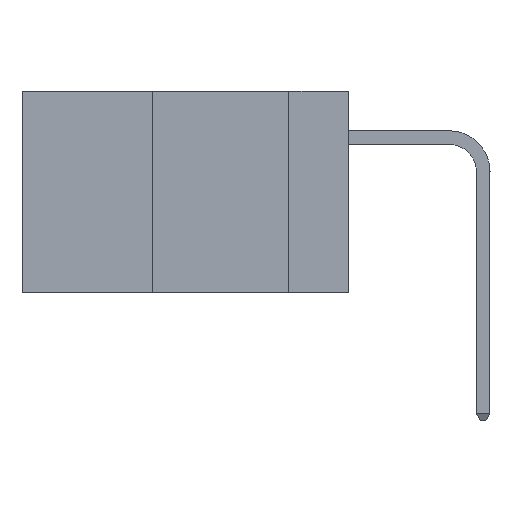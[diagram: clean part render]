
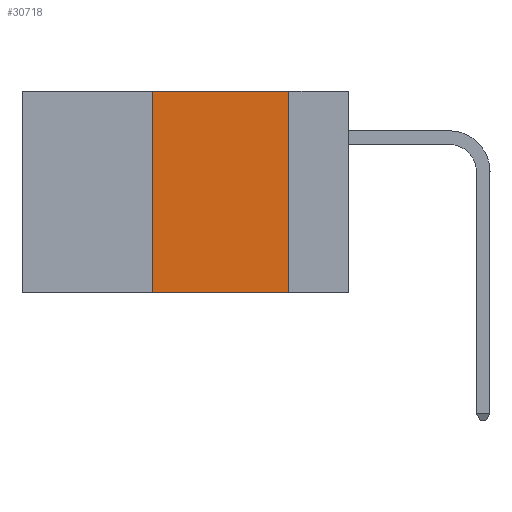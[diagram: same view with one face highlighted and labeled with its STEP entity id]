
A CAD part, left-side view. The second image highlights one B-rep face of the part: STEP entity #30718.
In plain terms, the highlighted planar face has unit normal (-1, 0, 0).
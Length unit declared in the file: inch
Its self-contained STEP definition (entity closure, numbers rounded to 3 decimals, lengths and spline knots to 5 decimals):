
#82 = CARTESIAN_POINT ( 'NONE',  ( 0., 0.11, 0. ) ) ;
#276 = DIRECTION ( 'NONE',  ( 0., 0., 1. ) ) ;
#2072 = CARTESIAN_POINT ( 'NONE',  ( 0., 0.11, 0. ) ) ;
#4077 = CARTESIAN_POINT ( 'NONE',  ( 0., 0.6, 0. ) ) ;
#4151 = ORIENTED_EDGE ( 'NONE', *, *, #21956, .F. ) ;
#4376 = CARTESIAN_POINT ( 'NONE',  ( 0., 0.6, -0.37 ) ) ;
#4894 = ORIENTED_EDGE ( 'NONE', *, *, #28098, .F. ) ;
#7425 = CARTESIAN_POINT ( 'NONE',  ( 0., 0.36, -0.37 ) ) ;
#9056 = DIRECTION ( 'NONE',  ( 0., 0., -1. ) ) ;
#9481 = CARTESIAN_POINT ( 'NONE',  ( 0., 0.6, 0. ) ) ;
#11064 = LINE ( 'NONE', #4077, #31831 ) ;
#12893 = ORIENTED_EDGE ( 'NONE', *, *, #17279, .T. ) ;
#13644 = VECTOR ( 'NONE', #29639, 39.37008 ) ;
#16273 = LINE ( 'NONE', #2072, #13644 ) ;
#17200 = DIRECTION ( 'NONE',  ( 0., -1., 0. ) ) ;
#17279 = EDGE_CURVE ( 'NONE', #19058, #21318, #33983, .T. ) ;
#17374 = VECTOR ( 'NONE', #276, 39.37008 ) ;
#18707 = VERTEX_POINT ( 'NONE', #35696 ) ;
#19058 = VERTEX_POINT ( 'NONE', #7425 ) ;
#21318 = VERTEX_POINT ( 'NONE', #23985 ) ;
#21956 = EDGE_CURVE ( 'NONE', #18707, #43145, #11064, .T. ) ;
#22112 = EDGE_CURVE ( 'NONE', #19058, #18707, #24281, .T. ) ;
#23985 = CARTESIAN_POINT ( 'NONE',  ( 0., 0.11, -0.37 ) ) ;
#24281 = LINE ( 'NONE', #31182, #17374 ) ;
#26159 = DIRECTION ( 'NONE',  ( 1., 0., 0. ) ) ;
#26860 = AXIS2_PLACEMENT_3D ( 'NONE', #9481, #26159, #9056 ) ;
#26951 = ORIENTED_EDGE ( 'NONE', *, *, #22112, .F. ) ;
#28098 = EDGE_CURVE ( 'NONE', #43145, #21318, #16273, .T. ) ;
#28211 = DIRECTION ( 'NONE',  ( 0., -1., 0. ) ) ;
#29639 = DIRECTION ( 'NONE',  ( 0., 0., -1. ) ) ;
#30718 = ADVANCED_FACE ( 'NONE', ( #34786 ), #42939, .F. ) ;
#31182 = CARTESIAN_POINT ( 'NONE',  ( 0., 0.36, 0. ) ) ;
#31831 = VECTOR ( 'NONE', #17200, 39.37008 ) ;
#33983 = LINE ( 'NONE', #4376, #43523 ) ;
#34786 = FACE_OUTER_BOUND ( 'NONE', #36191, .T. ) ;
#35696 = CARTESIAN_POINT ( 'NONE',  ( 0., 0.36, 0. ) ) ;
#36191 = EDGE_LOOP ( 'NONE', ( #4894, #4151, #26951, #12893 ) ) ;
#42939 = PLANE ( 'NONE',  #26860 ) ;
#43145 = VERTEX_POINT ( 'NONE', #82 ) ;
#43523 = VECTOR ( 'NONE', #28211, 39.37008 ) ;
